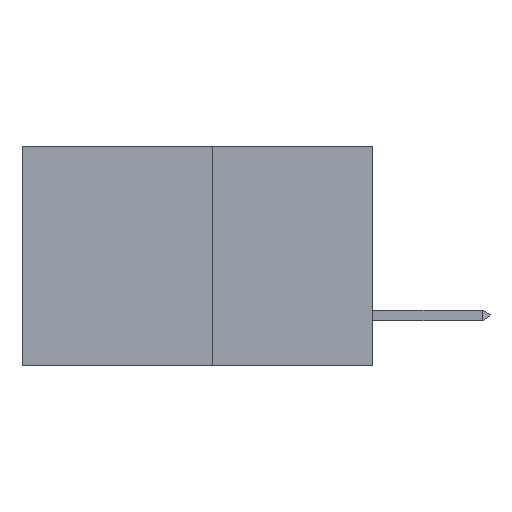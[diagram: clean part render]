
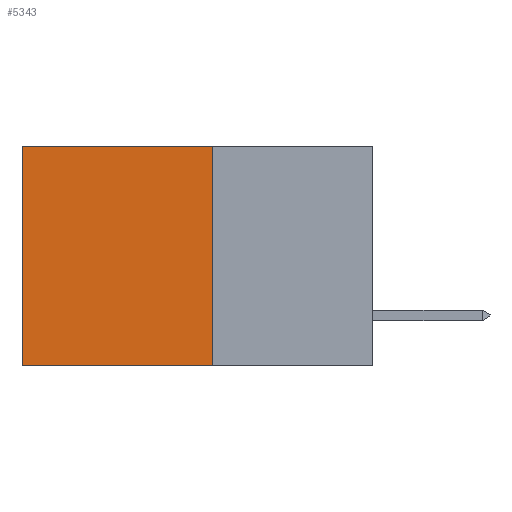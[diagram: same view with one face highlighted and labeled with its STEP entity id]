
A CAD part, left-side view. The second image highlights one B-rep face of the part: STEP entity #5343.
In plain terms, the highlighted planar face has unit normal (-1, 0, 0).
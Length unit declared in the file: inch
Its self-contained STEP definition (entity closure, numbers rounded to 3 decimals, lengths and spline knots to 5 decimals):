
#2178 = ORIENTED_EDGE ( 'NONE', *, *, #16997, .F. ) ;
#2739 = ORIENTED_EDGE ( 'NONE', *, *, #15114, .T. ) ;
#3045 = VERTEX_POINT ( 'NONE', #29155 ) ;
#3729 = DIRECTION ( 'NONE',  ( 0., 0., -1. ) ) ;
#3772 = DIRECTION ( 'NONE',  ( 1., 0., 0. ) ) ;
#4235 = CARTESIAN_POINT ( 'NONE',  ( 0.277, 0.27, -0.37 ) ) ;
#4972 = PLANE ( 'NONE',  #28021 ) ;
#5343 = ADVANCED_FACE ( 'NONE', ( #5371 ), #4972, .F. ) ;
#5371 = FACE_OUTER_BOUND ( 'NONE', #24392, .T. ) ;
#6808 = VERTEX_POINT ( 'NONE', #9655 ) ;
#7188 = CARTESIAN_POINT ( 'NONE',  ( 0.277, 0.27, 0. ) ) ;
#7833 = CARTESIAN_POINT ( 'NONE',  ( 0.277, 0.27, -0.37 ) ) ;
#9574 = VECTOR ( 'NONE', #21703, 39.37008 ) ;
#9655 = CARTESIAN_POINT ( 'NONE',  ( 0.277, 0.59, 0. ) ) ;
#10181 = VECTOR ( 'NONE', #11354, 39.37008 ) ;
#10444 = ORIENTED_EDGE ( 'NONE', *, *, #29442, .T. ) ;
#10922 = LINE ( 'NONE', #12193, #23241 ) ;
#11354 = DIRECTION ( 'NONE',  ( 0., 0., -1. ) ) ;
#12193 = CARTESIAN_POINT ( 'NONE',  ( 0.277, 0.27, -0.37 ) ) ;
#14676 = EDGE_CURVE ( 'NONE', #22000, #3045, #10922, .T. ) ;
#15114 = EDGE_CURVE ( 'NONE', #6808, #3045, #29310, .T. ) ;
#16404 = ORIENTED_EDGE ( 'NONE', *, *, #14676, .F. ) ;
#16457 = LINE ( 'NONE', #7833, #9574 ) ;
#16997 = EDGE_CURVE ( 'NONE', #26116, #22000, #16457, .T. ) ;
#17192 = VECTOR ( 'NONE', #25692, 39.37008 ) ;
#19576 = CARTESIAN_POINT ( 'NONE',  ( 0.277, 0.27, 0. ) ) ;
#21703 = DIRECTION ( 'NONE',  ( 0., 0., -1. ) ) ;
#22000 = VERTEX_POINT ( 'NONE', #23303 ) ;
#23241 = VECTOR ( 'NONE', #26036, 39.37008 ) ;
#23303 = CARTESIAN_POINT ( 'NONE',  ( 0.277, 0.27, -0.37 ) ) ;
#23312 = LINE ( 'NONE', #7188, #17192 ) ;
#24392 = EDGE_LOOP ( 'NONE', ( #2739, #16404, #2178, #10444 ) ) ;
#25222 = CARTESIAN_POINT ( 'NONE',  ( 0.277, 0.59, -0.37 ) ) ;
#25692 = DIRECTION ( 'NONE',  ( 0., 1., 0. ) ) ;
#26036 = DIRECTION ( 'NONE',  ( 0., 1., 0. ) ) ;
#26116 = VERTEX_POINT ( 'NONE', #19576 ) ;
#28021 = AXIS2_PLACEMENT_3D ( 'NONE', #4235, #3772, #3729 ) ;
#29155 = CARTESIAN_POINT ( 'NONE',  ( 0.277, 0.59, -0.37 ) ) ;
#29310 = LINE ( 'NONE', #25222, #10181 ) ;
#29442 = EDGE_CURVE ( 'NONE', #26116, #6808, #23312, .T. ) ;
